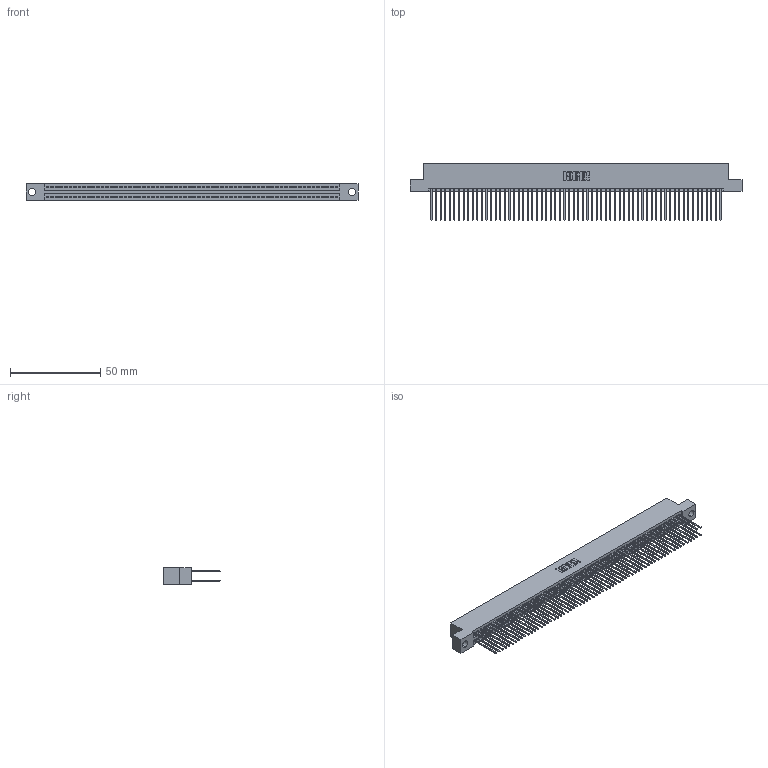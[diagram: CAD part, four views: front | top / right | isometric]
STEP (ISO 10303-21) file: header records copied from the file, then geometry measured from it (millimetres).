
FILE_DESCRIPTION (( 'STEP AP203' ), '1' );
FILE_NAME ('345-128-542-204.STEP', '2018-10-19T20:33:49', ( '' ), ( '' ), 'SwSTEP 2.0', 'SolidWorks 2016', '' );
FILE_SCHEMA (( 'CONFIG_CONTROL_DESIGN' ));
Length unit declared in the file: inch
Products named in the file (3): 345 Part_Flush Mounting Lugs - 0.156 Dia-TH; 345-128-542-204; 345-292-001_345-293-142
Assembly tree (129 placements, depth 2):
  345-128-542-204
    345 Part_Flush Mounting Lugs - 0.156 Dia-TH
    345-292-001_345-293-142  x128
Bounding box: 183.77 x 31.29 x 9.4 mm (x, y, z)
Volume: 18564.6 mm3; surface area: 30471.3 mm2
Topology: 129 solids, 129 shells, 6526 faces, 19413 edges, 12770 vertices
Faces by surface type: plane 4304, cylinder 2222
Entity records: 47275 total; most frequent: CARTESIAN_POINT 7904, ORIENTED_EDGE 7838, DIRECTION 6943, EDGE_CURVE 3919, VECTOR 3531, LINE 3531, VERTEX_POINT 2610, AXIS2_PLACEMENT_3D 1706
